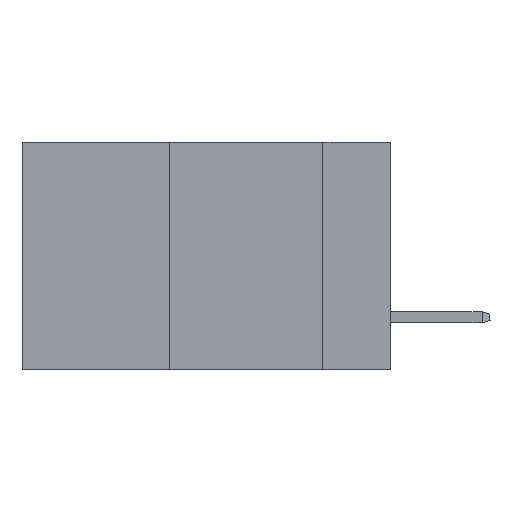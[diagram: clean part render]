
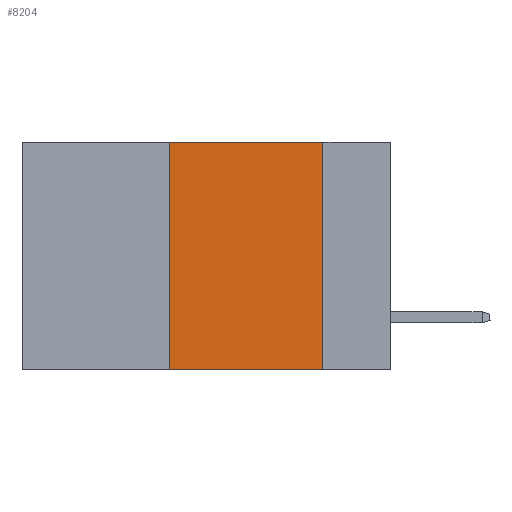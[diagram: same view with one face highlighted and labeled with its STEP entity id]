
A CAD part, left-side view. The second image highlights one B-rep face of the part: STEP entity #8204.
In plain terms, the highlighted planar face has unit normal (-1, 0, 0).
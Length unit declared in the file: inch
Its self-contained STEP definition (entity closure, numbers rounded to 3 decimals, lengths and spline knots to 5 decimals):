
#1322 = CARTESIAN_POINT ( 'NONE',  ( 0., 0.6, -0.37 ) ) ;
#1849 = CARTESIAN_POINT ( 'NONE',  ( 0., 0.6, 0. ) ) ;
#1885 = CARTESIAN_POINT ( 'NONE',  ( 0., 0.11, 0. ) ) ;
#2129 = LINE ( 'NONE', #7292, #12860 ) ;
#2718 = LINE ( 'NONE', #16322, #10627 ) ;
#2948 = PLANE ( 'NONE',  #6060 ) ;
#2972 = DIRECTION ( 'NONE',  ( 0., 0., 1. ) ) ;
#3034 = CARTESIAN_POINT ( 'NONE',  ( 0., 0.36, 0. ) ) ;
#3060 = ORIENTED_EDGE ( 'NONE', *, *, #12749, .F. ) ;
#3254 = EDGE_LOOP ( 'NONE', ( #4808, #3060, #8787, #6435 ) ) ;
#3531 = EDGE_CURVE ( 'NONE', #5452, #15230, #10240, .T. ) ;
#4808 = ORIENTED_EDGE ( 'NONE', *, *, #12861, .F. ) ;
#5452 = VERTEX_POINT ( 'NONE', #14821 ) ;
#5811 = DIRECTION ( 'NONE',  ( 0., 0., -1. ) ) ;
#6060 = AXIS2_PLACEMENT_3D ( 'NONE', #11426, #14266, #5811 ) ;
#6435 = ORIENTED_EDGE ( 'NONE', *, *, #3531, .T. ) ;
#7292 = CARTESIAN_POINT ( 'NONE',  ( 0., 0.36, 0. ) ) ;
#7311 = FACE_OUTER_BOUND ( 'NONE', #3254, .T. ) ;
#8204 = ADVANCED_FACE ( 'NONE', ( #7311 ), #2948, .F. ) ;
#8787 = ORIENTED_EDGE ( 'NONE', *, *, #11827, .F. ) ;
#10240 = LINE ( 'NONE', #1322, #11319 ) ;
#10508 = VERTEX_POINT ( 'NONE', #3034 ) ;
#10627 = VECTOR ( 'NONE', #16506, 39.37008 ) ;
#10850 = LINE ( 'NONE', #1849, #11066 ) ;
#11062 = DIRECTION ( 'NONE',  ( 0., -1., 0. ) ) ;
#11066 = VECTOR ( 'NONE', #14502, 39.37008 ) ;
#11319 = VECTOR ( 'NONE', #11062, 39.37008 ) ;
#11426 = CARTESIAN_POINT ( 'NONE',  ( 0., 0.6, 0. ) ) ;
#11827 = EDGE_CURVE ( 'NONE', #5452, #10508, #2129, .T. ) ;
#12749 = EDGE_CURVE ( 'NONE', #10508, #17381, #10850, .T. ) ;
#12860 = VECTOR ( 'NONE', #2972, 39.37008 ) ;
#12861 = EDGE_CURVE ( 'NONE', #17381, #15230, #2718, .T. ) ;
#14266 = DIRECTION ( 'NONE',  ( 1., 0., 0. ) ) ;
#14502 = DIRECTION ( 'NONE',  ( 0., -1., 0. ) ) ;
#14821 = CARTESIAN_POINT ( 'NONE',  ( 0., 0.36, -0.37 ) ) ;
#14980 = CARTESIAN_POINT ( 'NONE',  ( 0., 0.11, -0.37 ) ) ;
#15230 = VERTEX_POINT ( 'NONE', #14980 ) ;
#16322 = CARTESIAN_POINT ( 'NONE',  ( 0., 0.11, 0. ) ) ;
#16506 = DIRECTION ( 'NONE',  ( 0., 0., -1. ) ) ;
#17381 = VERTEX_POINT ( 'NONE', #1885 ) ;
